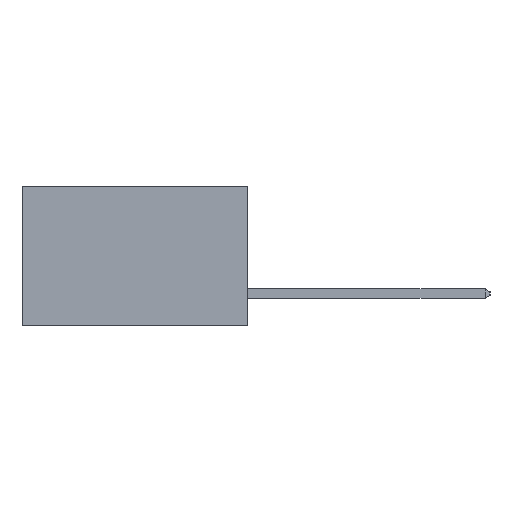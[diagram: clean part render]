
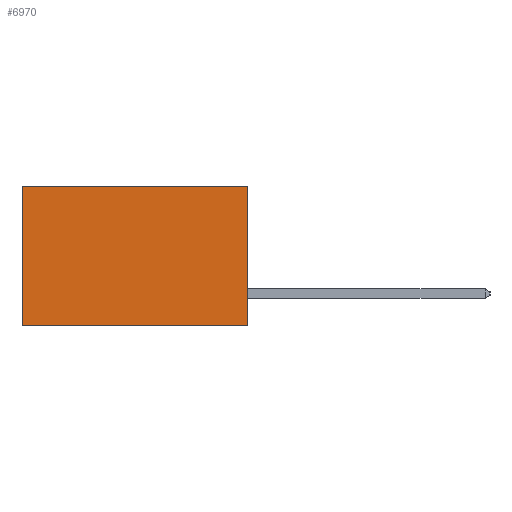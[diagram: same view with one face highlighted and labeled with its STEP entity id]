
A CAD part, left-side view. The second image highlights one B-rep face of the part: STEP entity #6970.
In plain terms, the highlighted planar face has unit normal (-1, 0, 0).
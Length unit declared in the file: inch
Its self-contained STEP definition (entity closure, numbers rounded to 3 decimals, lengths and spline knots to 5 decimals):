
#750 = DIRECTION ( 'NONE',  ( 0., 0., -1. ) ) ;
#946 = ORIENTED_EDGE ( 'NONE', *, *, #10831, .F. ) ;
#1196 = VECTOR ( 'NONE', #6560, 39.37008 ) ;
#2423 = CARTESIAN_POINT ( 'NONE',  ( 0.298, 0.6, -0.37 ) ) ;
#2468 = LINE ( 'NONE', #6160, #10672 ) ;
#2584 = LINE ( 'NONE', #12794, #8031 ) ;
#2846 = CARTESIAN_POINT ( 'NONE',  ( 0.298, 0.6, 0. ) ) ;
#2859 = DIRECTION ( 'NONE',  ( 0., 0., -1. ) ) ;
#3156 = EDGE_CURVE ( 'NONE', #5806, #9946, #2468, .T. ) ;
#3408 = DIRECTION ( 'NONE',  ( 1., 0., 0. ) ) ;
#3500 = EDGE_LOOP ( 'NONE', ( #9068, #946, #9915, #5841 ) ) ;
#3631 = VECTOR ( 'NONE', #11404, 39.37008 ) ;
#3779 = LINE ( 'NONE', #12816, #1196 ) ;
#4453 = CARTESIAN_POINT ( 'NONE',  ( 0.298, 0.6, 0. ) ) ;
#5480 = PLANE ( 'NONE',  #11321 ) ;
#5678 = EDGE_CURVE ( 'NONE', #5806, #8081, #2584, .T. ) ;
#5806 = VERTEX_POINT ( 'NONE', #11380 ) ;
#5841 = ORIENTED_EDGE ( 'NONE', *, *, #3156, .T. ) ;
#6058 = FACE_OUTER_BOUND ( 'NONE', #3500, .T. ) ;
#6111 = DIRECTION ( 'NONE',  ( 0., 1., 0. ) ) ;
#6160 = CARTESIAN_POINT ( 'NONE',  ( 0.298, 0., 0. ) ) ;
#6560 = DIRECTION ( 'NONE',  ( 0., 1., 0. ) ) ;
#6970 = ADVANCED_FACE ( 'NONE', ( #6058 ), #5480, .F. ) ;
#8031 = VECTOR ( 'NONE', #750, 39.37008 ) ;
#8081 = VERTEX_POINT ( 'NONE', #13061 ) ;
#8698 = VERTEX_POINT ( 'NONE', #2423 ) ;
#9068 = ORIENTED_EDGE ( 'NONE', *, *, #10635, .T. ) ;
#9711 = CARTESIAN_POINT ( 'NONE',  ( 0.298, 0., 0. ) ) ;
#9915 = ORIENTED_EDGE ( 'NONE', *, *, #5678, .F. ) ;
#9946 = VERTEX_POINT ( 'NONE', #4453 ) ;
#10635 = EDGE_CURVE ( 'NONE', #9946, #8698, #12090, .T. ) ;
#10672 = VECTOR ( 'NONE', #6111, 39.37008 ) ;
#10831 = EDGE_CURVE ( 'NONE', #8081, #8698, #3779, .T. ) ;
#11321 = AXIS2_PLACEMENT_3D ( 'NONE', #9711, #3408, #2859 ) ;
#11380 = CARTESIAN_POINT ( 'NONE',  ( 0.298, 0., 0. ) ) ;
#11404 = DIRECTION ( 'NONE',  ( 0., 0., -1. ) ) ;
#12090 = LINE ( 'NONE', #2846, #3631 ) ;
#12794 = CARTESIAN_POINT ( 'NONE',  ( 0.298, 0., 0. ) ) ;
#12816 = CARTESIAN_POINT ( 'NONE',  ( 0.298, 0., -0.37 ) ) ;
#13061 = CARTESIAN_POINT ( 'NONE',  ( 0.298, 0., -0.37 ) ) ;
